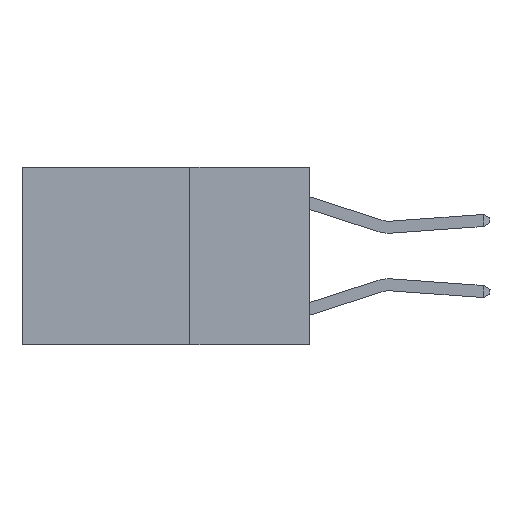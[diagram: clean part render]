
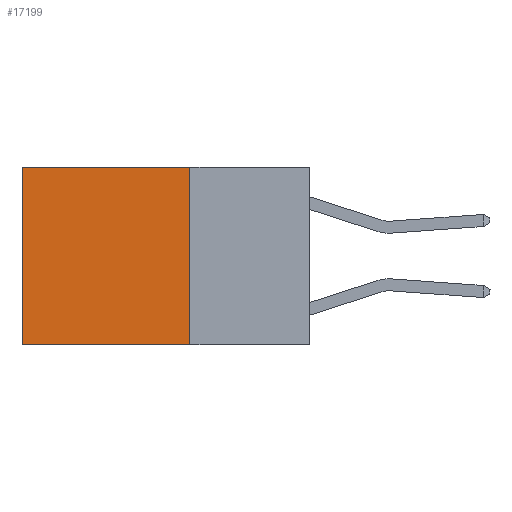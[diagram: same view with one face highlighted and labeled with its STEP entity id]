
A CAD part, left-side view. The second image highlights one B-rep face of the part: STEP entity #17199.
In plain terms, the highlighted planar face has unit normal (-1, 0, 0).
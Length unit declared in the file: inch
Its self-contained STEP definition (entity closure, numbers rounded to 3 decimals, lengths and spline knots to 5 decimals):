
#3039 = EDGE_CURVE ( 'NONE', #7236, #13882, #19240, .T. ) ;
#3379 = CARTESIAN_POINT ( 'NONE',  ( 0.2625, 0.6, 0. ) ) ;
#3400 = EDGE_CURVE ( 'NONE', #13882, #9145, #4922, .T. ) ;
#4119 = DIRECTION ( 'NONE',  ( 0., 1., 0. ) ) ;
#4399 = CARTESIAN_POINT ( 'NONE',  ( 0.2625, 0.25, -0.37 ) ) ;
#4553 = EDGE_CURVE ( 'NONE', #15626, #9145, #17874, .T. ) ;
#4922 = LINE ( 'NONE', #8003, #9190 ) ;
#7236 = VERTEX_POINT ( 'NONE', #15149 ) ;
#7322 = AXIS2_PLACEMENT_3D ( 'NONE', #11630, #8359, #13234 ) ;
#7460 = LINE ( 'NONE', #19575, #10520 ) ;
#7978 = ORIENTED_EDGE ( 'NONE', *, *, #3039, .T. ) ;
#8003 = CARTESIAN_POINT ( 'NONE',  ( 0.2625, 0.6, 0. ) ) ;
#8359 = DIRECTION ( 'NONE',  ( 1., 0., 0. ) ) ;
#8545 = FACE_OUTER_BOUND ( 'NONE', #11595, .T. ) ;
#9145 = VERTEX_POINT ( 'NONE', #18303 ) ;
#9175 = VECTOR ( 'NONE', #4119, 39.37008 ) ;
#9190 = VECTOR ( 'NONE', #14152, 39.37008 ) ;
#9658 = EDGE_CURVE ( 'NONE', #7236, #15626, #7460, .T. ) ;
#10520 = VECTOR ( 'NONE', #12017, 39.37008 ) ;
#11595 = EDGE_LOOP ( 'NONE', ( #19069, #19122, #12027, #7978 ) ) ;
#11630 = CARTESIAN_POINT ( 'NONE',  ( 0.2625, 0.25, 0. ) ) ;
#12017 = DIRECTION ( 'NONE',  ( 0., 0., -1. ) ) ;
#12027 = ORIENTED_EDGE ( 'NONE', *, *, #9658, .F. ) ;
#13234 = DIRECTION ( 'NONE',  ( 0., 0., -1. ) ) ;
#13882 = VERTEX_POINT ( 'NONE', #3379 ) ;
#14152 = DIRECTION ( 'NONE',  ( 0., 0., -1. ) ) ;
#14988 = CARTESIAN_POINT ( 'NONE',  ( 0.2625, 0.25, -0.37 ) ) ;
#15149 = CARTESIAN_POINT ( 'NONE',  ( 0.2625, 0.25, 0. ) ) ;
#15626 = VERTEX_POINT ( 'NONE', #4399 ) ;
#16055 = CARTESIAN_POINT ( 'NONE',  ( 0.2625, 0.25, 0. ) ) ;
#16109 = PLANE ( 'NONE',  #7322 ) ;
#17199 = ADVANCED_FACE ( 'NONE', ( #8545 ), #16109, .F. ) ;
#17874 = LINE ( 'NONE', #14988, #18312 ) ;
#18303 = CARTESIAN_POINT ( 'NONE',  ( 0.2625, 0.6, -0.37 ) ) ;
#18312 = VECTOR ( 'NONE', #19560, 39.37008 ) ;
#19069 = ORIENTED_EDGE ( 'NONE', *, *, #3400, .T. ) ;
#19122 = ORIENTED_EDGE ( 'NONE', *, *, #4553, .F. ) ;
#19240 = LINE ( 'NONE', #16055, #9175 ) ;
#19560 = DIRECTION ( 'NONE',  ( 0., 1., 0. ) ) ;
#19575 = CARTESIAN_POINT ( 'NONE',  ( 0.2625, 0.25, 0. ) ) ;
